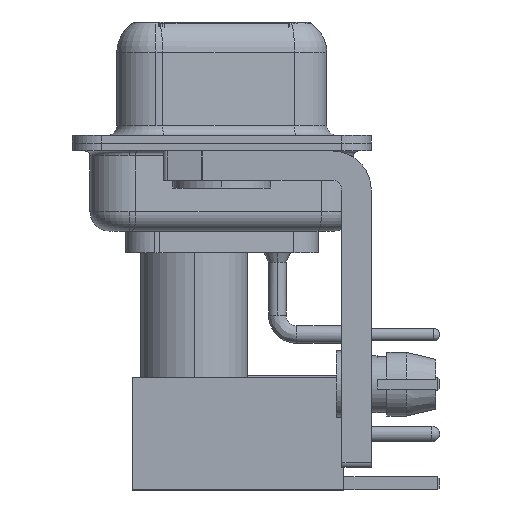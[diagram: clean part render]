
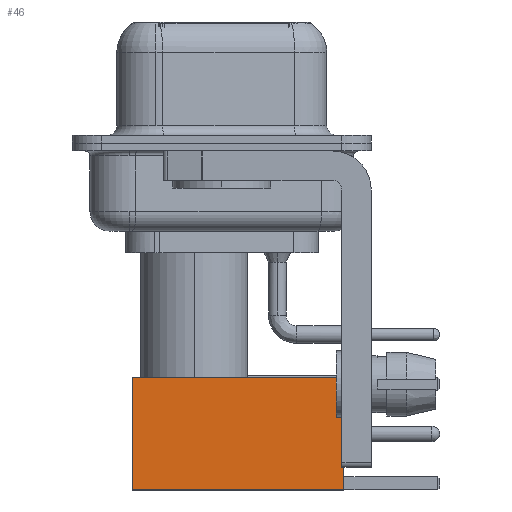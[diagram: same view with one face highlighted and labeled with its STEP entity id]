
A CAD part, left-side view. The second image highlights one B-rep face of the part: STEP entity #46.
In plain terms, the highlighted face is planar.
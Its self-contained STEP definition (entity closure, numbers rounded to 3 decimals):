
#46 = ADVANCED_FACE ( 'NONE', ( #3422 ), #33291, .T. ) ;
#367 = LINE ( 'NONE', #12189, #19062 ) ;
#882 = DIRECTION ( 'NONE',  ( 0., 1., 0. ) ) ;
#1385 = ORIENTED_EDGE ( 'NONE', *, *, #10063, .T. ) ;
#1574 = CARTESIAN_POINT ( 'NONE',  ( 2.875, 2.875, 0. ) ) ;
#2309 = EDGE_CURVE ( 'NONE', #35723, #25648, #8742, .T. ) ;
#3422 = FACE_OUTER_BOUND ( 'NONE', #34673, .T. ) ;
#3964 = VERTEX_POINT ( 'NONE', #18975 ) ;
#4142 = LINE ( 'NONE', #15955, #32351 ) ;
#5676 = EDGE_CURVE ( 'NONE', #23319, #3964, #367, .T. ) ;
#7430 = DIRECTION ( 'NONE',  ( 0., 0., -1. ) ) ;
#8202 = DIRECTION ( 'NONE',  ( 0., 0., -1. ) ) ;
#8742 = LINE ( 'NONE', #34953, #8848 ) ;
#8848 = VECTOR ( 'NONE', #38030, 1000. ) ;
#9079 = CARTESIAN_POINT ( 'NONE',  ( 2.875, 2.875, 10.82 ) ) ;
#10063 = EDGE_CURVE ( 'NONE', #23319, #35723, #11117, .T. ) ;
#11117 = LINE ( 'NONE', #22895, #13631 ) ;
#12189 = CARTESIAN_POINT ( 'NONE',  ( 0., 2.875, 10.82 ) ) ;
#12539 = DIRECTION ( 'NONE',  ( 0., 0., 1. ) ) ;
#13631 = VECTOR ( 'NONE', #8202, 1000. ) ;
#13924 = AXIS2_PLACEMENT_3D ( 'NONE', #29775, #882, #12539 ) ;
#15277 = DIRECTION ( 'NONE',  ( -1., 0., 0. ) ) ;
#15955 = CARTESIAN_POINT ( 'NONE',  ( -2.875, 2.875, 0. ) ) ;
#18975 = CARTESIAN_POINT ( 'NONE',  ( -2.875, 2.875, 10.82 ) ) ;
#19062 = VECTOR ( 'NONE', #15277, 1000. ) ;
#20792 = EDGE_CURVE ( 'NONE', #3964, #25648, #4142, .T. ) ;
#22895 = CARTESIAN_POINT ( 'NONE',  ( 2.875, 2.875, 0. ) ) ;
#23319 = VERTEX_POINT ( 'NONE', #9079 ) ;
#25625 = CARTESIAN_POINT ( 'NONE',  ( -2.875, 2.875, 0. ) ) ;
#25648 = VERTEX_POINT ( 'NONE', #25625 ) ;
#29775 = CARTESIAN_POINT ( 'NONE',  ( 2.875, 2.875, 0. ) ) ;
#31351 = ORIENTED_EDGE ( 'NONE', *, *, #2309, .T. ) ;
#32351 = VECTOR ( 'NONE', #7430, 1000. ) ;
#33291 = PLANE ( 'NONE',  #13924 ) ;
#33416 = ORIENTED_EDGE ( 'NONE', *, *, #5676, .F. ) ;
#34673 = EDGE_LOOP ( 'NONE', ( #1385, #31351, #36340, #33416 ) ) ;
#34953 = CARTESIAN_POINT ( 'NONE',  ( 0., 2.875, 0. ) ) ;
#35723 = VERTEX_POINT ( 'NONE', #1574 ) ;
#36340 = ORIENTED_EDGE ( 'NONE', *, *, #20792, .F. ) ;
#38030 = DIRECTION ( 'NONE',  ( -1., 0., 0. ) ) ;
